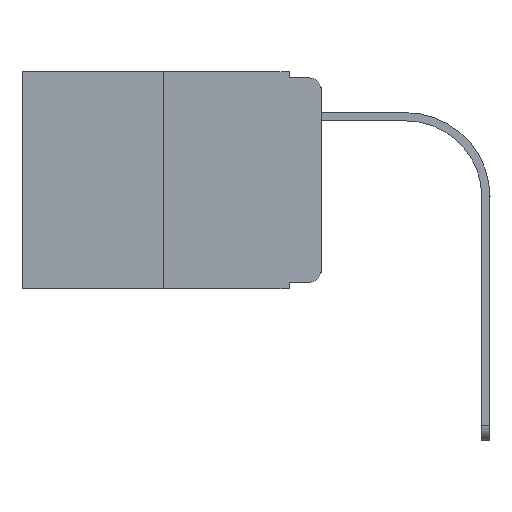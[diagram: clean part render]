
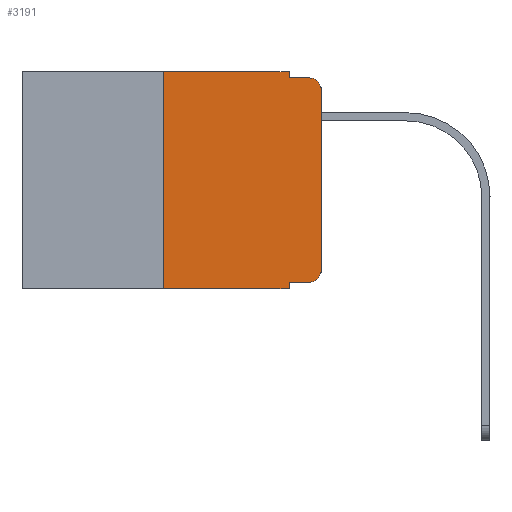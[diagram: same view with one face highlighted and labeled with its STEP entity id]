
A CAD part, left-side view. The second image highlights one B-rep face of the part: STEP entity #3191.
In plain terms, the highlighted planar face has unit normal (-1, 0, 0).
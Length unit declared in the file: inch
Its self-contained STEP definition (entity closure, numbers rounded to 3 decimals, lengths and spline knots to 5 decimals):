
#247 = CARTESIAN_POINT ( 'NONE',  ( 0., 0.02, -0.333 ) ) ;
#325 = ORIENTED_EDGE ( 'NONE', *, *, #4615, .F. ) ;
#380 = VECTOR ( 'NONE', #3206, 39.37008 ) ;
#391 = CARTESIAN_POINT ( 'NONE',  ( 0., 0.051, -0.01 ) ) ;
#491 = DIRECTION ( 'NONE',  ( 0., 0., -1. ) ) ;
#534 = ORIENTED_EDGE ( 'NONE', *, *, #5450, .F. ) ;
#575 = DIRECTION ( 'NONE',  ( 0., -1., 0. ) ) ;
#884 = CARTESIAN_POINT ( 'NONE',  ( 0., 0., -0.03 ) ) ;
#979 = LINE ( 'NONE', #4915, #11387 ) ;
#1122 = CARTESIAN_POINT ( 'NONE',  ( 0., 0.02, -0.313 ) ) ;
#1243 = CARTESIAN_POINT ( 'NONE',  ( 0., 0.051, -0.333 ) ) ;
#1302 = DIRECTION ( 'NONE',  ( 0., 0., -1. ) ) ;
#1487 = VERTEX_POINT ( 'NONE', #9114 ) ;
#1637 = DIRECTION ( 'NONE',  ( 0., -1., 0. ) ) ;
#1752 = DIRECTION ( 'NONE',  ( 1., 0., 0. ) ) ;
#1819 = CARTESIAN_POINT ( 'NONE',  ( 0., 0.473, -0.343 ) ) ;
#2029 = VERTEX_POINT ( 'NONE', #247 ) ;
#2445 = VERTEX_POINT ( 'NONE', #10061 ) ;
#3010 = VERTEX_POINT ( 'NONE', #391 ) ;
#3191 = ADVANCED_FACE ( 'NONE', ( #7787 ), #7591, .F. ) ;
#3205 = CARTESIAN_POINT ( 'NONE',  ( 0., 0.25, 0. ) ) ;
#3206 = DIRECTION ( 'NONE',  ( 0., 0., -1. ) ) ;
#3354 = VERTEX_POINT ( 'NONE', #5881 ) ;
#3401 = LINE ( 'NONE', #3205, #12452 ) ;
#3594 = LINE ( 'NONE', #11600, #13033 ) ;
#3664 = LINE ( 'NONE', #7661, #12694 ) ;
#3677 = VERTEX_POINT ( 'NONE', #884 ) ;
#3718 = VECTOR ( 'NONE', #575, 39.37008 ) ;
#3920 = VERTEX_POINT ( 'NONE', #5108 ) ;
#4227 = ORIENTED_EDGE ( 'NONE', *, *, #6878, .T. ) ;
#4520 = LINE ( 'NONE', #7481, #3718 ) ;
#4615 = EDGE_CURVE ( 'NONE', #3010, #5085, #4520, .T. ) ;
#4915 = CARTESIAN_POINT ( 'NONE',  ( 0., 0.473, 0. ) ) ;
#5085 = VERTEX_POINT ( 'NONE', #10393 ) ;
#5108 = CARTESIAN_POINT ( 'NONE',  ( 0., 0.25, 0. ) ) ;
#5233 = CARTESIAN_POINT ( 'NONE',  ( 0., 0.02, -0.03 ) ) ;
#5372 = DIRECTION ( 'NONE',  ( 0., 0., 1. ) ) ;
#5450 = EDGE_CURVE ( 'NONE', #3354, #7266, #3594, .T. ) ;
#5742 = EDGE_LOOP ( 'NONE', ( #12292, #9475, #325, #10519, #8312, #11361, #8442, #534, #9691, #4227 ) ) ;
#5855 = VECTOR ( 'NONE', #1637, 39.37008 ) ;
#5881 = CARTESIAN_POINT ( 'NONE',  ( 0., 0.051, -0.333 ) ) ;
#6228 = CIRCLE ( 'NONE', #12822, 0.02 ) ;
#6655 = CIRCLE ( 'NONE', #11527, 0.02 ) ;
#6692 = LINE ( 'NONE', #1819, #5855 ) ;
#6878 = EDGE_CURVE ( 'NONE', #2029, #10486, #6655, .T. ) ;
#6890 = DIRECTION ( 'NONE',  ( 0., -1., 0. ) ) ;
#7079 = LINE ( 'NONE', #7150, #380 ) ;
#7150 = CARTESIAN_POINT ( 'NONE',  ( 0., 0.051, 0. ) ) ;
#7266 = VERTEX_POINT ( 'NONE', #8058 ) ;
#7384 = EDGE_CURVE ( 'NONE', #3677, #5085, #6228, .T. ) ;
#7392 = CARTESIAN_POINT ( 'NONE',  ( 0., 0., -0.313 ) ) ;
#7481 = CARTESIAN_POINT ( 'NONE',  ( 0., 0.051, -0.01 ) ) ;
#7591 = PLANE ( 'NONE',  #9521 ) ;
#7661 = CARTESIAN_POINT ( 'NONE',  ( 0., 0., 0. ) ) ;
#7730 = DIRECTION ( 'NONE',  ( 0., 0., 1. ) ) ;
#7787 = FACE_OUTER_BOUND ( 'NONE', #5742, .T. ) ;
#8058 = CARTESIAN_POINT ( 'NONE',  ( 0., 0.051, -0.343 ) ) ;
#8312 = ORIENTED_EDGE ( 'NONE', *, *, #10026, .F. ) ;
#8332 = DIRECTION ( 'NONE',  ( 0., -1., 0. ) ) ;
#8379 = VECTOR ( 'NONE', #8332, 39.37008 ) ;
#8442 = ORIENTED_EDGE ( 'NONE', *, *, #12826, .T. ) ;
#8563 = EDGE_CURVE ( 'NONE', #3354, #2029, #12401, .T. ) ;
#8674 = EDGE_CURVE ( 'NONE', #2445, #3010, #7079, .T. ) ;
#9114 = CARTESIAN_POINT ( 'NONE',  ( 0., 0.25, -0.343 ) ) ;
#9292 = DIRECTION ( 'NONE',  ( 0., 0., -1. ) ) ;
#9475 = ORIENTED_EDGE ( 'NONE', *, *, #7384, .T. ) ;
#9521 = AXIS2_PLACEMENT_3D ( 'NONE', #9724, #1752, #11662 ) ;
#9691 = ORIENTED_EDGE ( 'NONE', *, *, #8563, .T. ) ;
#9724 = CARTESIAN_POINT ( 'NONE',  ( 0., 0.473, 0. ) ) ;
#10026 = EDGE_CURVE ( 'NONE', #3920, #2445, #979, .T. ) ;
#10061 = CARTESIAN_POINT ( 'NONE',  ( 0., 0.051, 0. ) ) ;
#10091 = EDGE_CURVE ( 'NONE', #1487, #3920, #3401, .T. ) ;
#10274 = DIRECTION ( 'NONE',  ( -1., 0., 0. ) ) ;
#10316 = DIRECTION ( 'NONE',  ( -1., 0., 0. ) ) ;
#10393 = CARTESIAN_POINT ( 'NONE',  ( 0., 0.02, -0.01 ) ) ;
#10486 = VERTEX_POINT ( 'NONE', #7392 ) ;
#10519 = ORIENTED_EDGE ( 'NONE', *, *, #8674, .F. ) ;
#11361 = ORIENTED_EDGE ( 'NONE', *, *, #10091, .F. ) ;
#11387 = VECTOR ( 'NONE', #6890, 39.37008 ) ;
#11518 = EDGE_CURVE ( 'NONE', #10486, #3677, #3664, .T. ) ;
#11527 = AXIS2_PLACEMENT_3D ( 'NONE', #1122, #10274, #9292 ) ;
#11600 = CARTESIAN_POINT ( 'NONE',  ( 0., 0.051, 0. ) ) ;
#11662 = DIRECTION ( 'NONE',  ( 0., 0., -1. ) ) ;
#12292 = ORIENTED_EDGE ( 'NONE', *, *, #11518, .T. ) ;
#12401 = LINE ( 'NONE', #1243, #8379 ) ;
#12452 = VECTOR ( 'NONE', #5372, 39.37008 ) ;
#12694 = VECTOR ( 'NONE', #7730, 39.37008 ) ;
#12822 = AXIS2_PLACEMENT_3D ( 'NONE', #5233, #10316, #1302 ) ;
#12826 = EDGE_CURVE ( 'NONE', #1487, #7266, #6692, .T. ) ;
#13033 = VECTOR ( 'NONE', #491, 39.37008 ) ;
